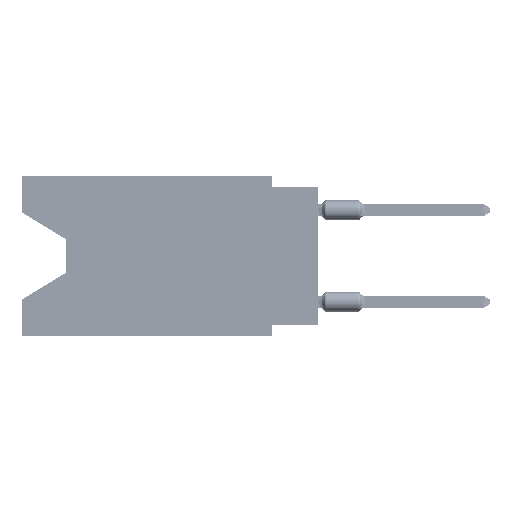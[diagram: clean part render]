
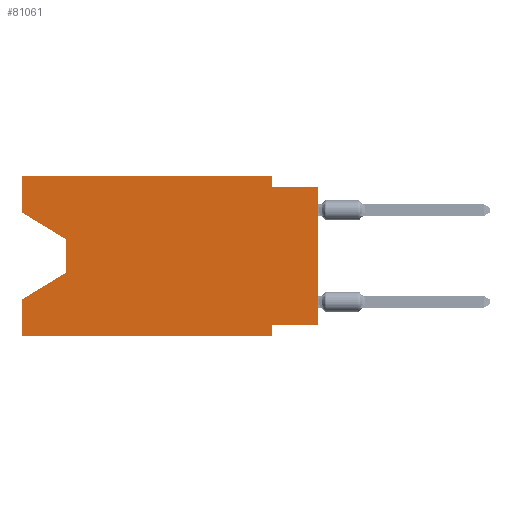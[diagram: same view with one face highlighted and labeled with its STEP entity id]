
A CAD part, left-side view. The second image highlights one B-rep face of the part: STEP entity #81061.
In plain terms, the highlighted planar face has unit normal (-1, 0, 0).
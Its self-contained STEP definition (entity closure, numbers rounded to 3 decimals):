
#2607 = VECTOR ( 'NONE', #28161, 1000. ) ;
#4421 = CARTESIAN_POINT ( 'NONE',  ( 0., 0., -8.255 ) ) ;
#4422 = DIRECTION ( 'NONE',  ( 0., 0., 1. ) ) ;
#5212 = VERTEX_POINT ( 'NONE', #75104 ) ;
#5896 = ORIENTED_EDGE ( 'NONE', *, *, #21598, .F. ) ;
#5923 = CARTESIAN_POINT ( 'NONE',  ( 0., 16.383, -6.852 ) ) ;
#6391 = VERTEX_POINT ( 'NONE', #29292 ) ;
#6993 = VECTOR ( 'NONE', #55092, 1000. ) ;
#7100 = CARTESIAN_POINT ( 'NONE',  ( 0., 13.97, -5.385 ) ) ;
#7236 = ORIENTED_EDGE ( 'NONE', *, *, #61404, .F. ) ;
#8134 = VECTOR ( 'NONE', #64604, 1000. ) ;
#9527 = ORIENTED_EDGE ( 'NONE', *, *, #60798, .F. ) ;
#9973 = PLANE ( 'NONE',  #40590 ) ;
#10135 = DIRECTION ( 'NONE',  ( 0., 0.855, -0.519 ) ) ;
#11695 = LINE ( 'NONE', #30960, #47176 ) ;
#11955 = CARTESIAN_POINT ( 'NONE',  ( 0., 2.54, 0. ) ) ;
#12367 = CARTESIAN_POINT ( 'NONE',  ( 0., 13.97, -3.505 ) ) ;
#16120 = CARTESIAN_POINT ( 'NONE',  ( 0., 13.97, -5.385 ) ) ;
#16434 = DIRECTION ( 'NONE',  ( 0., 0., -1. ) ) ;
#16715 = LINE ( 'NONE', #43249, #28576 ) ;
#18698 = ORIENTED_EDGE ( 'NONE', *, *, #19181, .T. ) ;
#19181 = EDGE_CURVE ( 'NONE', #66042, #77379, #57755, .T. ) ;
#19989 = CARTESIAN_POINT ( 'NONE',  ( 0., 2.54, 0. ) ) ;
#21598 = EDGE_CURVE ( 'NONE', #65655, #45594, #48986, .T. ) ;
#22138 = LINE ( 'NONE', #16120, #48298 ) ;
#22821 = DIRECTION ( 'NONE',  ( 0., 0., -1. ) ) ;
#23813 = VERTEX_POINT ( 'NONE', #5923 ) ;
#24185 = VECTOR ( 'NONE', #62245, 1000. ) ;
#24408 = CARTESIAN_POINT ( 'NONE',  ( 0., 2.54, -8.89 ) ) ;
#24782 = VERTEX_POINT ( 'NONE', #19989 ) ;
#25346 = EDGE_LOOP ( 'NONE', ( #76496, #18698, #43653, #57179, #42959, #5896, #81163, #35100, #9527, #44961, #7236, #80511 ) ) ;
#26762 = CARTESIAN_POINT ( 'NONE',  ( 0., 0., -0.635 ) ) ;
#27913 = VECTOR ( 'NONE', #38060, 1000. ) ;
#28057 = CARTESIAN_POINT ( 'NONE',  ( 0., 16.383, 0. ) ) ;
#28161 = DIRECTION ( 'NONE',  ( 0., 0., 1. ) ) ;
#28450 = EDGE_CURVE ( 'NONE', #59578, #45594, #16715, .T. ) ;
#28576 = VECTOR ( 'NONE', #56116, 1000. ) ;
#29292 = CARTESIAN_POINT ( 'NONE',  ( 0., 2.54, -0.635 ) ) ;
#30474 = EDGE_CURVE ( 'NONE', #59706, #66042, #34962, .T. ) ;
#30960 = CARTESIAN_POINT ( 'NONE',  ( 0., 0., 0. ) ) ;
#31797 = EDGE_CURVE ( 'NONE', #77379, #23813, #22138, .T. ) ;
#34962 = LINE ( 'NONE', #54668, #6993 ) ;
#35100 = ORIENTED_EDGE ( 'NONE', *, *, #35517, .T. ) ;
#35517 = EDGE_CURVE ( 'NONE', #5212, #37422, #11695, .T. ) ;
#37422 = VERTEX_POINT ( 'NONE', #26762 ) ;
#37436 = LINE ( 'NONE', #63552, #69511 ) ;
#37711 = EDGE_CURVE ( 'NONE', #5212, #65655, #49399, .T. ) ;
#38060 = DIRECTION ( 'NONE',  ( 0., 0., -1. ) ) ;
#40590 = AXIS2_PLACEMENT_3D ( 'NONE', #42491, #40814, #22821 ) ;
#40814 = DIRECTION ( 'NONE',  ( 1., 0., 0. ) ) ;
#42491 = CARTESIAN_POINT ( 'NONE',  ( 0., 16.383, 0. ) ) ;
#42959 = ORIENTED_EDGE ( 'NONE', *, *, #28450, .T. ) ;
#43249 = CARTESIAN_POINT ( 'NONE',  ( 0., 16.383, -8.89 ) ) ;
#43653 = ORIENTED_EDGE ( 'NONE', *, *, #31797, .T. ) ;
#43934 = VECTOR ( 'NONE', #16434, 1000. ) ;
#44961 = ORIENTED_EDGE ( 'NONE', *, *, #48293, .F. ) ;
#45594 = VERTEX_POINT ( 'NONE', #24408 ) ;
#46390 = CARTESIAN_POINT ( 'NONE',  ( 0., 13.97, -3.505 ) ) ;
#47166 = DIRECTION ( 'NONE',  ( 0., 0., 1. ) ) ;
#47176 = VECTOR ( 'NONE', #4422, 1000. ) ;
#48293 = EDGE_CURVE ( 'NONE', #24782, #6391, #70617, .T. ) ;
#48298 = VECTOR ( 'NONE', #10135, 1000. ) ;
#48986 = LINE ( 'NONE', #75100, #43934 ) ;
#49083 = VECTOR ( 'NONE', #79674, 1000. ) ;
#49127 = CARTESIAN_POINT ( 'NONE',  ( 0., 16.383, -8.89 ) ) ;
#49399 = LINE ( 'NONE', #4421, #24185 ) ;
#51543 = DIRECTION ( 'NONE',  ( 0., -1., 0. ) ) ;
#53449 = LINE ( 'NONE', #79156, #2607 ) ;
#54577 = EDGE_CURVE ( 'NONE', #59578, #23813, #78892, .T. ) ;
#54668 = CARTESIAN_POINT ( 'NONE',  ( 0., 16.383, -2.038 ) ) ;
#55092 = DIRECTION ( 'NONE',  ( 0., -0.855, -0.519 ) ) ;
#56116 = DIRECTION ( 'NONE',  ( 0., -1., 0. ) ) ;
#57179 = ORIENTED_EDGE ( 'NONE', *, *, #54577, .F. ) ;
#57755 = LINE ( 'NONE', #12367, #8134 ) ;
#59578 = VERTEX_POINT ( 'NONE', #49127 ) ;
#59611 = CARTESIAN_POINT ( 'NONE',  ( 0., 16.383, 0. ) ) ;
#59706 = VERTEX_POINT ( 'NONE', #66492 ) ;
#59771 = CARTESIAN_POINT ( 'NONE',  ( 0., 2.54, -8.255 ) ) ;
#60798 = EDGE_CURVE ( 'NONE', #6391, #37422, #37436, .T. ) ;
#61404 = EDGE_CURVE ( 'NONE', #77500, #24782, #71562, .T. ) ;
#62245 = DIRECTION ( 'NONE',  ( 0., 1., 0. ) ) ;
#63552 = CARTESIAN_POINT ( 'NONE',  ( 0., 0., -0.635 ) ) ;
#64604 = DIRECTION ( 'NONE',  ( 0., 0., -1. ) ) ;
#65655 = VERTEX_POINT ( 'NONE', #59771 ) ;
#66042 = VERTEX_POINT ( 'NONE', #46390 ) ;
#66492 = CARTESIAN_POINT ( 'NONE',  ( 0., 16.383, -2.038 ) ) ;
#69511 = VECTOR ( 'NONE', #51543, 1000. ) ;
#69738 = EDGE_CURVE ( 'NONE', #59706, #77500, #53449, .T. ) ;
#70617 = LINE ( 'NONE', #11955, #27913 ) ;
#71562 = LINE ( 'NONE', #71978, #49083 ) ;
#71978 = CARTESIAN_POINT ( 'NONE',  ( 0., 16.383, 0. ) ) ;
#75100 = CARTESIAN_POINT ( 'NONE',  ( 0., 2.54, -8.89 ) ) ;
#75104 = CARTESIAN_POINT ( 'NONE',  ( 0., 0., -8.255 ) ) ;
#76496 = ORIENTED_EDGE ( 'NONE', *, *, #30474, .T. ) ;
#77379 = VERTEX_POINT ( 'NONE', #7100 ) ;
#77500 = VERTEX_POINT ( 'NONE', #28057 ) ;
#78418 = VECTOR ( 'NONE', #47166, 1000. ) ;
#78892 = LINE ( 'NONE', #59611, #78418 ) ;
#79156 = CARTESIAN_POINT ( 'NONE',  ( 0., 16.383, 0. ) ) ;
#79674 = DIRECTION ( 'NONE',  ( 0., -1., 0. ) ) ;
#80221 = FACE_OUTER_BOUND ( 'NONE', #25346, .T. ) ;
#80511 = ORIENTED_EDGE ( 'NONE', *, *, #69738, .F. ) ;
#81061 = ADVANCED_FACE ( 'NONE', ( #80221 ), #9973, .F. ) ;
#81163 = ORIENTED_EDGE ( 'NONE', *, *, #37711, .F. ) ;
